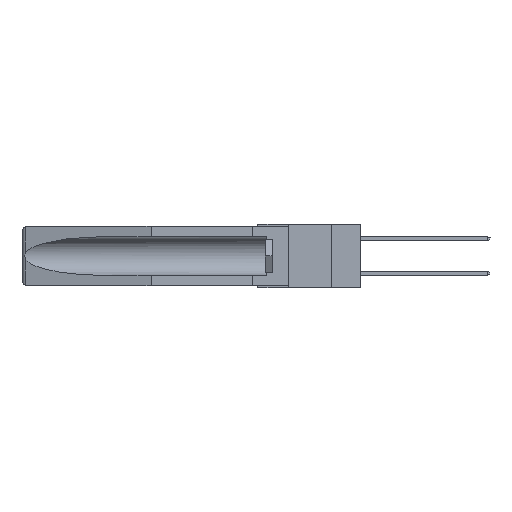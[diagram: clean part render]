
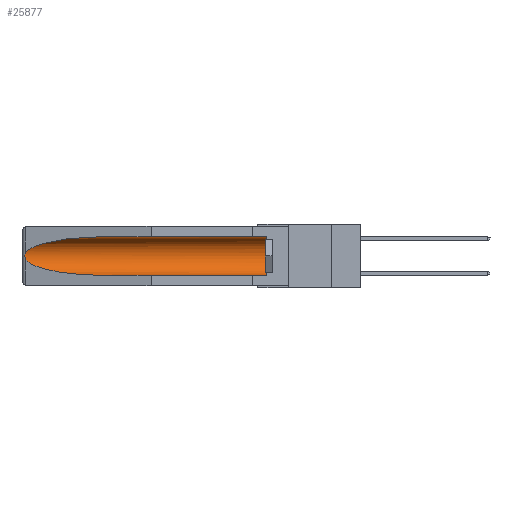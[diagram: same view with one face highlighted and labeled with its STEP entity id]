
A CAD part, left-side view. The second image highlights one B-rep face of the part: STEP entity #25877.
In plain terms, the highlighted cylindrical face has radius 2.857 mm (diameter 5.715 mm), a partial arc.
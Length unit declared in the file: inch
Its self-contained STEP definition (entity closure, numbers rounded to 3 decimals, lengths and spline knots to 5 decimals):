
#627 = VERTEX_POINT ( 'NONE', #21424 ) ;
#827 = CARTESIAN_POINT ( 'NONE',  ( 0.155, -0.30754, -0.059 ) ) ;
#1172 = CARTESIAN_POINT ( 'NONE',  ( 0.26537, 1.52718, -0.19328 ) ) ;
#1409 = CARTESIAN_POINT ( 'NONE',  ( 0.26537, 1.52718, -0.19328 ) ) ;
#1866 = DIRECTION ( 'NONE',  ( 0., 0., 1. ) ) ;
#2272 = VERTEX_POINT ( 'NONE', #4765 ) ;
#2496 = CARTESIAN_POINT ( 'NONE',  ( 0.155, 0.126, -0.284 ) ) ;
#3321 = EDGE_CURVE ( 'NONE', #18745, #22863, #27009, .T. ) ;
#4056 = DIRECTION ( 'NONE',  ( 0., 1., 0. ) ) ;
#4192 = CARTESIAN_POINT ( 'NONE',  ( 0.155, 1.07973, -0.284 ) ) ;
#4216 = FACE_OUTER_BOUND ( 'NONE', #27347, .T. ) ;
#4642 = EDGE_CURVE ( 'NONE', #18745, #8666, #23666, .T. ) ;
#4648 = DIRECTION ( 'NONE',  ( 0., 1., 0. ) ) ;
#4765 = CARTESIAN_POINT ( 'NONE',  ( 0.155, 1.07973, -0.059 ) ) ;
#5061 = AXIS2_PLACEMENT_3D ( 'NONE', #28512, #4648, #1866 ) ;
#5188 = CARTESIAN_POINT ( 'NONE',  ( 0.155, 0.126, -0.1715 ) ) ;
#5840 = CARTESIAN_POINT ( 'NONE',  ( 0.2675, 1.53308, -0.16763 ) ) ;
#6221 = DIRECTION ( 'NONE',  ( 0., 1., 0. ) ) ;
#7079 = CARTESIAN_POINT ( 'NONE',  ( 0.155, 1.07973, -0.059 ) ) ;
#7258 = VERTEX_POINT ( 'NONE', #1409 ) ;
#8164 = CARTESIAN_POINT ( 'NONE',  ( 0.2673, 1.53269, -0.17917 ) ) ;
#8258 =( BOUNDED_CURVE ( )  B_SPLINE_CURVE ( 3, ( #7079, #16418, #31071, #18626 ),
 .UNSPECIFIED., .F., .T. ) 
 B_SPLINE_CURVE_WITH_KNOTS ( ( 4, 4 ),
 ( 4.71239, 6.08839 ),
 .UNSPECIFIED. ) 
 CURVE ( )  GEOMETRIC_REPRESENTATION_ITEM ( )  RATIONAL_B_SPLINE_CURVE ( ( 1., 0.848, 0.848, 1. ) ) 
 REPRESENTATION_ITEM ( '' )  );
#8402 = DIRECTION ( 'NONE',  ( 0., 0., 1. ) ) ;
#8666 = VERTEX_POINT ( 'NONE', #4192 ) ;
#8692 = CARTESIAN_POINT ( 'NONE',  ( 0.155, 1.07973, -0.284 ) ) ;
#8986 = ORIENTED_EDGE ( 'NONE', *, *, #4642, .F. ) ;
#10053 = ORIENTED_EDGE ( 'NONE', *, *, #20526, .T. ) ;
#12702 = CARTESIAN_POINT ( 'NONE',  ( 0.26597, 1.52961, -0.15275 ) ) ;
#13207 = CARTESIAN_POINT ( 'NONE',  ( 0.26654, 1.53092, -0.15636 ) ) ;
#13673 = ORIENTED_EDGE ( 'NONE', *, *, #14816, .T. ) ;
#14390 = CARTESIAN_POINT ( 'NONE',  ( 0.155, 0.126, -0.059 ) ) ;
#14564 = EDGE_CURVE ( 'NONE', #627, #7258, #30757, .T. ) ;
#14816 = EDGE_CURVE ( 'NONE', #22863, #2272, #27425, .T. ) ;
#15298 = CARTESIAN_POINT ( 'NONE',  ( 0.26537, 1.52718, -0.14972 ) ) ;
#16361 = ORIENTED_EDGE ( 'NONE', *, *, #3321, .T. ) ;
#16418 = CARTESIAN_POINT ( 'NONE',  ( 0.21114, 1.30732, -0.059 ) ) ;
#18252 = CARTESIAN_POINT ( 'NONE',  ( 0.25451, 1.48313, -0.24835 ) ) ;
#18626 = CARTESIAN_POINT ( 'NONE',  ( 0.26537, 1.52718, -0.14972 ) ) ;
#18745 = VERTEX_POINT ( 'NONE', #2496 ) ;
#20438 = AXIS2_PLACEMENT_3D ( 'NONE', #5188, #24431, #8402 ) ;
#20526 = EDGE_CURVE ( 'NONE', #2272, #627, #8258, .T. ) ;
#20687 = CARTESIAN_POINT ( 'NONE',  ( 0.21114, 1.30732, -0.284 ) ) ;
#20816 =( BOUNDED_CURVE ( )  B_SPLINE_CURVE ( 3, ( #20900, #18252, #20687, #8692 ),
 .UNSPECIFIED., .F., .F. ) 
 B_SPLINE_CURVE_WITH_KNOTS ( ( 4, 4 ),
 ( 0.1948, 1.5708 ),
 .UNSPECIFIED. ) 
 CURVE ( )  GEOMETRIC_REPRESENTATION_ITEM ( )  RATIONAL_B_SPLINE_CURVE ( ( 1., 0.848, 0.848, 1. ) ) 
 REPRESENTATION_ITEM ( '' )  );
#20900 = CARTESIAN_POINT ( 'NONE',  ( 0.26537, 1.52718, -0.19328 ) ) ;
#21424 = CARTESIAN_POINT ( 'NONE',  ( 0.26537, 1.52718, -0.14972 ) ) ;
#22592 = CARTESIAN_POINT ( 'NONE',  ( 0.2675, 1.53308, -0.17534 ) ) ;
#22810 = CARTESIAN_POINT ( 'NONE',  ( 0.26597, 1.5296, -0.19026 ) ) ;
#22863 = VERTEX_POINT ( 'NONE', #14390 ) ;
#23666 = LINE ( 'NONE', #28022, #24066 ) ;
#24066 = VECTOR ( 'NONE', #4056, 39.37008 ) ;
#24431 = DIRECTION ( 'NONE',  ( 0., -1., 0. ) ) ;
#25024 = CARTESIAN_POINT ( 'NONE',  ( 0.2673, 1.5327, -0.16383 ) ) ;
#25877 = ADVANCED_FACE ( 'NONE', ( #4216 ), #27232, .F. ) ;
#26270 = VECTOR ( 'NONE', #6221, 39.37008 ) ;
#26301 = ORIENTED_EDGE ( 'NONE', *, *, #14564, .T. ) ;
#27009 = CIRCLE ( 'NONE', #20438, 0.1125 ) ;
#27232 = CYLINDRICAL_SURFACE ( 'NONE', #5061, 0.1125 ) ;
#27347 = EDGE_LOOP ( 'NONE', ( #10053, #26301, #29327, #8986, #16361, #13673 ) ) ;
#27425 = LINE ( 'NONE', #827, #26270 ) ;
#27701 = CARTESIAN_POINT ( 'NONE',  ( 0.26655, 1.53094, -0.18657 ) ) ;
#28022 = CARTESIAN_POINT ( 'NONE',  ( 0.155, -0.30754, -0.284 ) ) ;
#28051 = EDGE_CURVE ( 'NONE', #7258, #8666, #20816, .T. ) ;
#28512 = CARTESIAN_POINT ( 'NONE',  ( 0.155, -0.30754, -0.1715 ) ) ;
#29327 = ORIENTED_EDGE ( 'NONE', *, *, #28051, .T. ) ;
#30757 = B_SPLINE_CURVE_WITH_KNOTS ( 'NONE', 3,
 ( #15298, #12702, #13207, #25024, #5840, #22592, #8164, #27701, #22810, #1172 ),
 .UNSPECIFIED., .F., .F.,
 ( 4, 2, 2, 2, 4 ),
 ( 0., 0.00029, 0.00058, 0.00087, 0.00117 ),
 .UNSPECIFIED. ) ;
#31071 = CARTESIAN_POINT ( 'NONE',  ( 0.25451, 1.48313, -0.09465 ) ) ;
